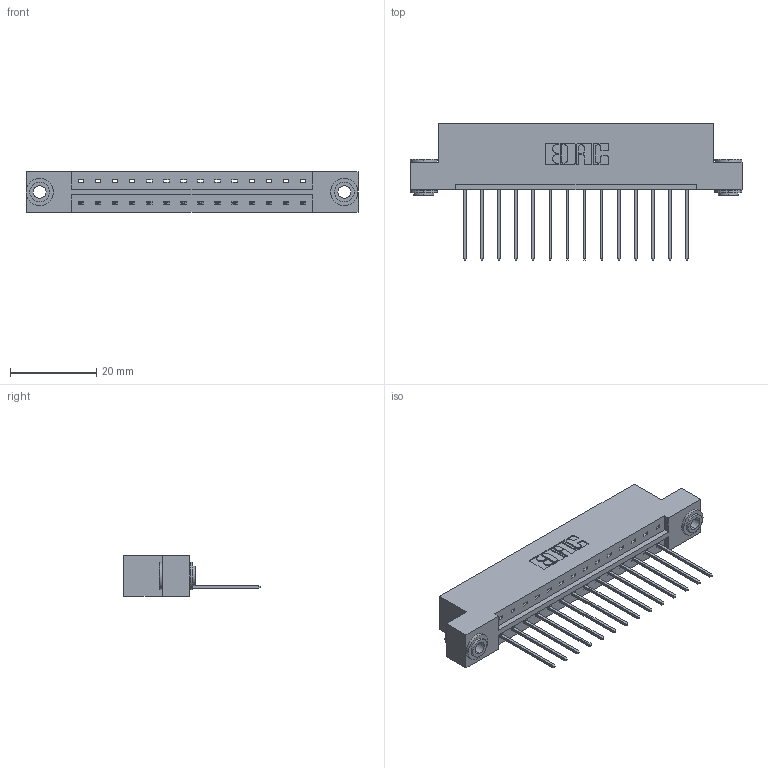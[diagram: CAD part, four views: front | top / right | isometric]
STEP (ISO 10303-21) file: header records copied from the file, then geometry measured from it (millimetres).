
FILE_DESCRIPTION (( 'STEP AP203' ), '1' );
FILE_NAME ('833-014-542-103.STEP', '2020-05-31T14:10:12', ( '' ), ( '' ), 'SwSTEP 2.0', 'SolidWorks 2020', '' );
FILE_SCHEMA (( 'CONFIG_CONTROL_DESIGN' ));
Length unit declared in the file: inch
Products named in the file (4): 833-014-542-103; 345-292-001_345-293-142; 833 Part_Flush - .156 Dia - TH; 345-250-002_345-250-002-102
Assembly tree (17 placements, depth 2):
  833-014-542-103
    833 Part_Flush - .156 Dia - TH
    345-292-001_345-293-142  x14
    345-250-002_345-250-002-102  x2
Bounding box: 77.01 x 31.63 x 9.4 mm (x, y, z)
Volume: 7559.4 mm3; surface area: 8428.5 mm2
Topology: 17 solids, 17 shells, 964 faces, 2851 edges, 1878 vertices
Faces by surface type: plane 668, cylinder 288, cone 8
Entity records: 12848 total; most frequent: CARTESIAN_POINT 2199, ORIENTED_EDGE 2142, DIRECTION 1945, EDGE_CURVE 1071, LINE 919, VECTOR 919, VERTEX_POINT 710, AXIS2_PLACEMENT_3D 513
